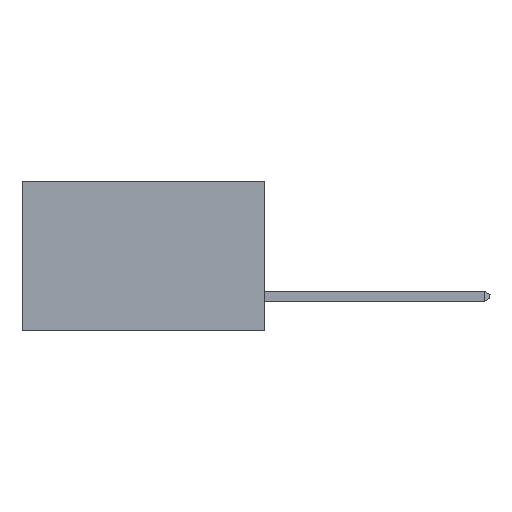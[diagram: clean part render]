
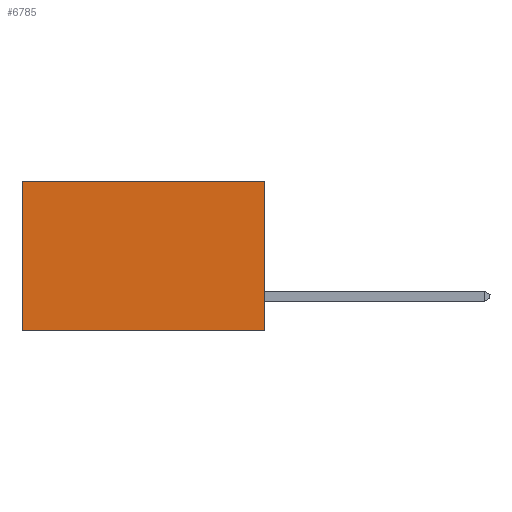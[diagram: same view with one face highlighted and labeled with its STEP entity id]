
A CAD part, left-side view. The second image highlights one B-rep face of the part: STEP entity #6785.
In plain terms, the highlighted planar face has unit normal (-1, 0, 0).
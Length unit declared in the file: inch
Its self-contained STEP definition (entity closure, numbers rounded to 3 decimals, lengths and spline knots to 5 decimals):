
#21 = PLANE ( 'NONE',  #1909 ) ;
#1111 = CARTESIAN_POINT ( 'NONE',  ( 0.2615, 0.6, 0. ) ) ;
#1909 = AXIS2_PLACEMENT_3D ( 'NONE', #8253, #9776, #13142 ) ;
#2646 = EDGE_LOOP ( 'NONE', ( #4829, #10666, #2797, #7184 ) ) ;
#2797 = ORIENTED_EDGE ( 'NONE', *, *, #12902, .F. ) ;
#3421 = VECTOR ( 'NONE', #15689, 39.37008 ) ;
#3822 = VERTEX_POINT ( 'NONE', #11691 ) ;
#4569 = LINE ( 'NONE', #9439, #9565 ) ;
#4829 = ORIENTED_EDGE ( 'NONE', *, *, #15082, .T. ) ;
#5018 = LINE ( 'NONE', #15039, #5705 ) ;
#5421 = CARTESIAN_POINT ( 'NONE',  ( 0.2615, 0., 0. ) ) ;
#5659 = VECTOR ( 'NONE', #9467, 39.37008 ) ;
#5705 = VECTOR ( 'NONE', #9887, 39.37008 ) ;
#6089 = EDGE_CURVE ( 'NONE', #9448, #9007, #5018, .T. ) ;
#6785 = ADVANCED_FACE ( 'NONE', ( #7125 ), #21, .F. ) ;
#7125 = FACE_OUTER_BOUND ( 'NONE', #2646, .T. ) ;
#7184 = ORIENTED_EDGE ( 'NONE', *, *, #6089, .T. ) ;
#7246 = EDGE_CURVE ( 'NONE', #7957, #3822, #4569, .T. ) ;
#7957 = VERTEX_POINT ( 'NONE', #15221 ) ;
#8032 = LINE ( 'NONE', #15616, #5659 ) ;
#8253 = CARTESIAN_POINT ( 'NONE',  ( 0.2615, 0., -0.37 ) ) ;
#9007 = VERTEX_POINT ( 'NONE', #1111 ) ;
#9439 = CARTESIAN_POINT ( 'NONE',  ( 0.2615, 0., -0.37 ) ) ;
#9448 = VERTEX_POINT ( 'NONE', #5421 ) ;
#9467 = DIRECTION ( 'NONE',  ( 0., 0., -1. ) ) ;
#9565 = VECTOR ( 'NONE', #14310, 39.37008 ) ;
#9776 = DIRECTION ( 'NONE',  ( 1., 0., 0. ) ) ;
#9887 = DIRECTION ( 'NONE',  ( 0., 1., 0. ) ) ;
#10666 = ORIENTED_EDGE ( 'NONE', *, *, #7246, .F. ) ;
#10671 = CARTESIAN_POINT ( 'NONE',  ( 0.2615, 0.6, -0.37 ) ) ;
#11691 = CARTESIAN_POINT ( 'NONE',  ( 0.2615, 0.6, -0.37 ) ) ;
#12902 = EDGE_CURVE ( 'NONE', #9448, #7957, #8032, .T. ) ;
#13142 = DIRECTION ( 'NONE',  ( 0., 0., -1. ) ) ;
#13220 = LINE ( 'NONE', #10671, #3421 ) ;
#14310 = DIRECTION ( 'NONE',  ( 0., 1., 0. ) ) ;
#15039 = CARTESIAN_POINT ( 'NONE',  ( 0.2615, 0., 0. ) ) ;
#15082 = EDGE_CURVE ( 'NONE', #9007, #3822, #13220, .T. ) ;
#15221 = CARTESIAN_POINT ( 'NONE',  ( 0.2615, 0., -0.37 ) ) ;
#15616 = CARTESIAN_POINT ( 'NONE',  ( 0.2615, 0., -0.37 ) ) ;
#15689 = DIRECTION ( 'NONE',  ( 0., 0., -1. ) ) ;
